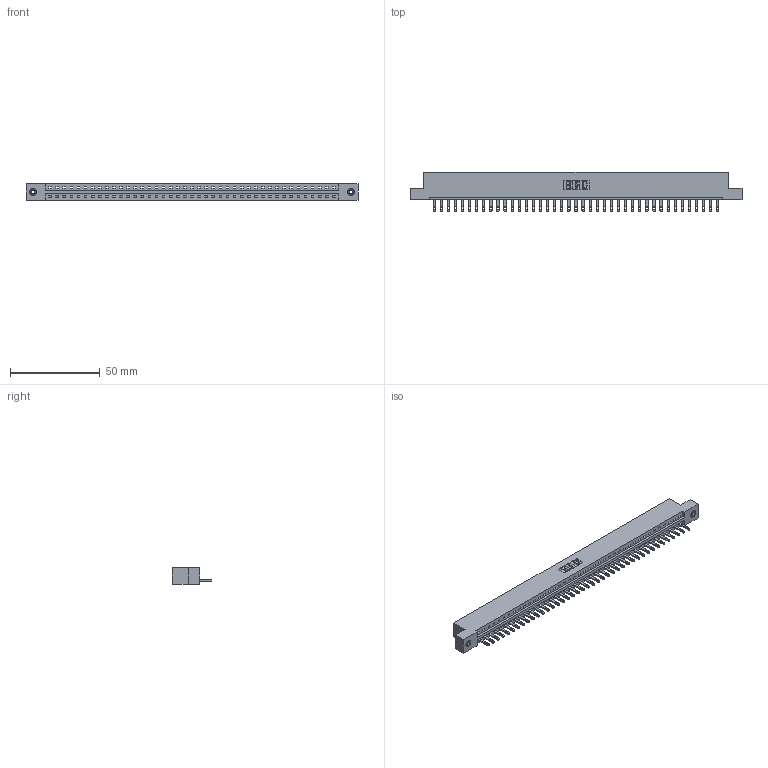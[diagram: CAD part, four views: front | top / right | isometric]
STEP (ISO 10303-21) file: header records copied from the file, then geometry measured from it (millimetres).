
FILE_DESCRIPTION (( 'STEP AP203' ), '1' );
FILE_NAME ('887-041-500-108.STEP', '2020-09-20T23:42:00', ( '' ), ( '' ), 'SwSTEP 2.0', 'SolidWorks 2020', '' );
FILE_SCHEMA (( 'CONFIG_CONTROL_DESIGN' ));
Length unit declared in the file: inch
Products named in the file (4): 345-292-001_345-293-100; 837 Part_Flush Mounting Lugs - 0.156 Dia-TI; 345-250-001_345-250-003-102; 887-041-500-108
Assembly tree (44 placements, depth 2):
  887-041-500-108
    837 Part_Flush Mounting Lugs - 0.156 Dia-TI
    345-292-001_345-293-100  x41
    345-250-001_345-250-003-102  x2
Bounding box: 185.47 x 21.85 x 9.4 mm (x, y, z)
Volume: 19282.9 mm3; surface area: 20045.9 mm2
Topology: 44 solids, 44 shells, 2552 faces, 7827 edges, 5210 vertices
Faces by surface type: plane 1742, cylinder 794, cone 12, torus 4
Entity records: 31722 total; most frequent: CARTESIAN_POINT 5504, ORIENTED_EDGE 5474, DIRECTION 4669, EDGE_CURVE 2737, LINE 2585, VECTOR 2585, VERTEX_POINT 1820, AXIS2_PLACEMENT_3D 1042
